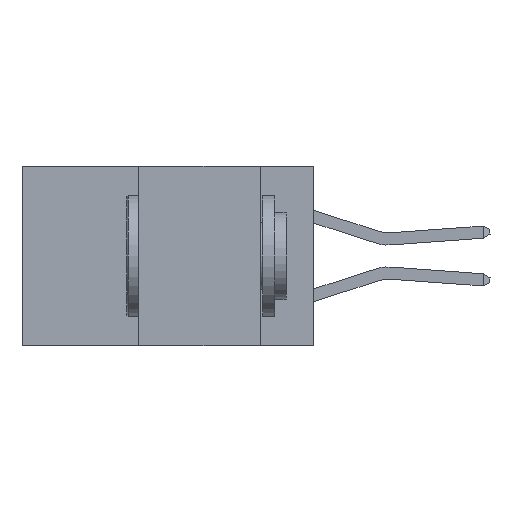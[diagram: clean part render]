
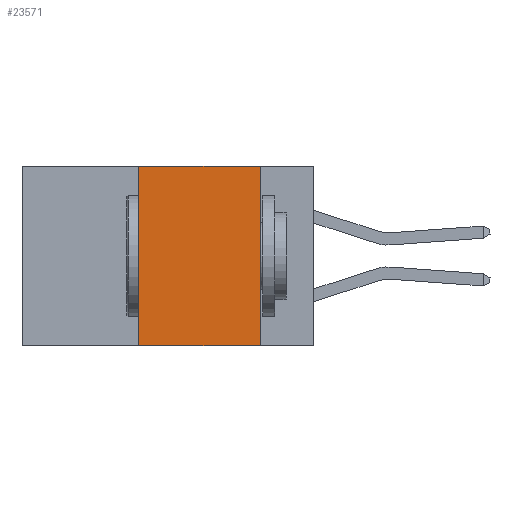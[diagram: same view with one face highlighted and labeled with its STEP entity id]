
A CAD part, left-side view. The second image highlights one B-rep face of the part: STEP entity #23571.
In plain terms, the highlighted planar face has unit normal (-1, 0, 0).
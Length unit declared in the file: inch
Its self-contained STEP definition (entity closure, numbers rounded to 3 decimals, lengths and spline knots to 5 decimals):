
#4555 = VERTEX_POINT ( 'NONE', #36466 ) ;
#5603 = VECTOR ( 'NONE', #31926, 39.37008 ) ;
#7573 = EDGE_CURVE ( 'NONE', #28701, #41625, #14828, .T. ) ;
#7772 = EDGE_CURVE ( 'NONE', #4555, #41625, #32672, .T. ) ;
#8424 = CARTESIAN_POINT ( 'NONE',  ( 0., 0.6, 0. ) ) ;
#8743 = CARTESIAN_POINT ( 'NONE',  ( 0., 0.6, -0.37 ) ) ;
#9219 = PLANE ( 'NONE',  #38251 ) ;
#11197 = CARTESIAN_POINT ( 'NONE',  ( 0., 0.11, 0. ) ) ;
#12417 = CARTESIAN_POINT ( 'NONE',  ( 0., 0.36, 0. ) ) ;
#14828 = LINE ( 'NONE', #11197, #5603 ) ;
#16197 = CARTESIAN_POINT ( 'NONE',  ( 0., 0.6, 0. ) ) ;
#18359 = ORIENTED_EDGE ( 'NONE', *, *, #40065, .F. ) ;
#19659 = DIRECTION ( 'NONE',  ( 0., 0., -1. ) ) ;
#23197 = CARTESIAN_POINT ( 'NONE',  ( 0., 0.11, -0.37 ) ) ;
#23464 = VECTOR ( 'NONE', #39936, 39.37008 ) ;
#23571 = ADVANCED_FACE ( 'NONE', ( #29984 ), #9219, .F. ) ;
#23823 = VECTOR ( 'NONE', #43087, 39.37008 ) ;
#24293 = ORIENTED_EDGE ( 'NONE', *, *, #7573, .F. ) ;
#26868 = LINE ( 'NONE', #12417, #44190 ) ;
#28701 = VERTEX_POINT ( 'NONE', #38516 ) ;
#29777 = ORIENTED_EDGE ( 'NONE', *, *, #7772, .T. ) ;
#29984 = FACE_OUTER_BOUND ( 'NONE', #42082, .T. ) ;
#30003 = VERTEX_POINT ( 'NONE', #31120 ) ;
#31120 = CARTESIAN_POINT ( 'NONE',  ( 0., 0.36, 0. ) ) ;
#31367 = ORIENTED_EDGE ( 'NONE', *, *, #42188, .F. ) ;
#31926 = DIRECTION ( 'NONE',  ( 0., 0., -1. ) ) ;
#32672 = LINE ( 'NONE', #8743, #23464 ) ;
#33022 = LINE ( 'NONE', #8424, #23823 ) ;
#36466 = CARTESIAN_POINT ( 'NONE',  ( 0., 0.36, -0.37 ) ) ;
#38251 = AXIS2_PLACEMENT_3D ( 'NONE', #16197, #40397, #19659 ) ;
#38516 = CARTESIAN_POINT ( 'NONE',  ( 0., 0.11, 0. ) ) ;
#39936 = DIRECTION ( 'NONE',  ( 0., -1., 0. ) ) ;
#40065 = EDGE_CURVE ( 'NONE', #30003, #28701, #33022, .T. ) ;
#40397 = DIRECTION ( 'NONE',  ( 1., 0., 0. ) ) ;
#41625 = VERTEX_POINT ( 'NONE', #23197 ) ;
#42082 = EDGE_LOOP ( 'NONE', ( #24293, #18359, #31367, #29777 ) ) ;
#42188 = EDGE_CURVE ( 'NONE', #4555, #30003, #26868, .T. ) ;
#43087 = DIRECTION ( 'NONE',  ( 0., -1., 0. ) ) ;
#43588 = DIRECTION ( 'NONE',  ( 0., 0., 1. ) ) ;
#44190 = VECTOR ( 'NONE', #43588, 39.37008 ) ;
